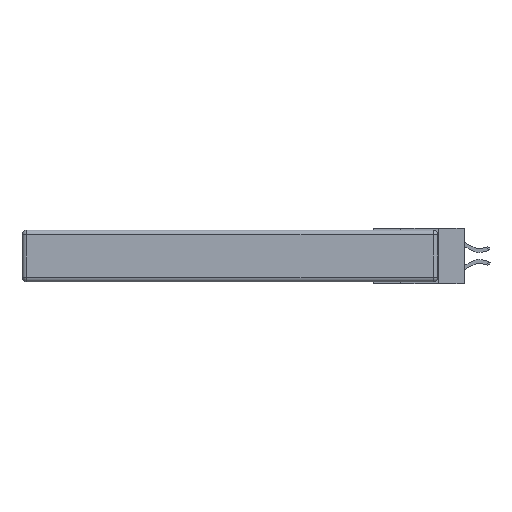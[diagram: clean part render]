
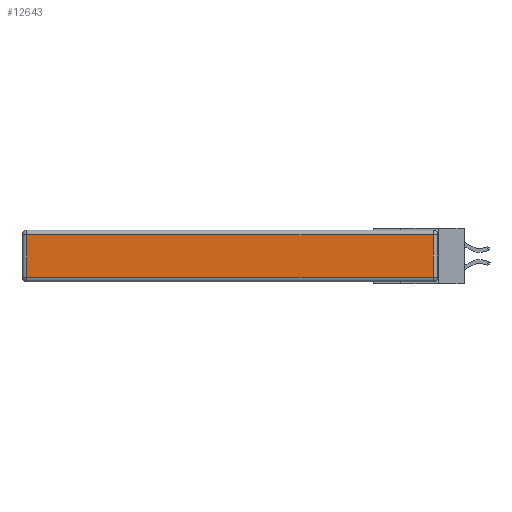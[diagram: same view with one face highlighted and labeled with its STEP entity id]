
A CAD part, left-side view. The second image highlights one B-rep face of the part: STEP entity #12643.
In plain terms, the highlighted planar face has unit normal (-1, 0, 0).
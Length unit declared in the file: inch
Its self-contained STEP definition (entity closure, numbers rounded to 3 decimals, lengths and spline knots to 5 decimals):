
#684 = CARTESIAN_POINT ( 'NONE',  ( 0., 2.72, -0.343 ) ) ;
#1159 = VECTOR ( 'NONE', #8741, 39.37008 ) ;
#1696 = CARTESIAN_POINT ( 'NONE',  ( 0., 0., -0.313 ) ) ;
#1807 = CARTESIAN_POINT ( 'NONE',  ( 0., 2.75, -0.03 ) ) ;
#2645 = ORIENTED_EDGE ( 'NONE', *, *, #13484, .T. ) ;
#2786 = DIRECTION ( 'NONE',  ( 0., 0., -1. ) ) ;
#3207 = CARTESIAN_POINT ( 'NONE',  ( 0., 0.03, -0.343 ) ) ;
#4506 = ORIENTED_EDGE ( 'NONE', *, *, #6585, .T. ) ;
#4867 = DIRECTION ( 'NONE',  ( 0., -1., 0. ) ) ;
#6332 = EDGE_CURVE ( 'NONE', #13808, #13094, #7221, .T. ) ;
#6565 = EDGE_CURVE ( 'NONE', #13094, #7169, #8097, .T. ) ;
#6585 = EDGE_CURVE ( 'NONE', #7169, #8328, #13773, .T. ) ;
#6616 = DIRECTION ( 'NONE',  ( -1., 0., 0. ) ) ;
#6771 = VECTOR ( 'NONE', #4867, 39.37008 ) ;
#7148 = ORIENTED_EDGE ( 'NONE', *, *, #6332, .T. ) ;
#7169 = VERTEX_POINT ( 'NONE', #9755 ) ;
#7221 = LINE ( 'NONE', #3207, #1159 ) ;
#8097 = LINE ( 'NONE', #1807, #10703 ) ;
#8328 = VERTEX_POINT ( 'NONE', #11223 ) ;
#8741 = DIRECTION ( 'NONE',  ( 0., 0., 1. ) ) ;
#9755 = CARTESIAN_POINT ( 'NONE',  ( 0., 2.72, -0.03 ) ) ;
#9903 = CARTESIAN_POINT ( 'NONE',  ( 0., 0., -0.343 ) ) ;
#10002 = DIRECTION ( 'NONE',  ( 0., 0., 1. ) ) ;
#10081 = PLANE ( 'NONE',  #13512 ) ;
#10699 = DIRECTION ( 'NONE',  ( 0., 1., 0. ) ) ;
#10703 = VECTOR ( 'NONE', #10699, 39.37008 ) ;
#11223 = CARTESIAN_POINT ( 'NONE',  ( 0., 2.72, -0.313 ) ) ;
#11753 = VECTOR ( 'NONE', #2786, 39.37008 ) ;
#12005 = LINE ( 'NONE', #1696, #6771 ) ;
#12018 = FACE_OUTER_BOUND ( 'NONE', #13466, .T. ) ;
#12643 = ADVANCED_FACE ( 'NONE', ( #12018 ), #10081, .T. ) ;
#12677 = ORIENTED_EDGE ( 'NONE', *, *, #6565, .T. ) ;
#12812 = CARTESIAN_POINT ( 'NONE',  ( 0., 0.03, -0.03 ) ) ;
#12817 = CARTESIAN_POINT ( 'NONE',  ( 0., 0.03, -0.313 ) ) ;
#13094 = VERTEX_POINT ( 'NONE', #12812 ) ;
#13466 = EDGE_LOOP ( 'NONE', ( #2645, #7148, #12677, #4506 ) ) ;
#13484 = EDGE_CURVE ( 'NONE', #8328, #13808, #12005, .T. ) ;
#13512 = AXIS2_PLACEMENT_3D ( 'NONE', #9903, #6616, #10002 ) ;
#13773 = LINE ( 'NONE', #684, #11753 ) ;
#13808 = VERTEX_POINT ( 'NONE', #12817 ) ;
